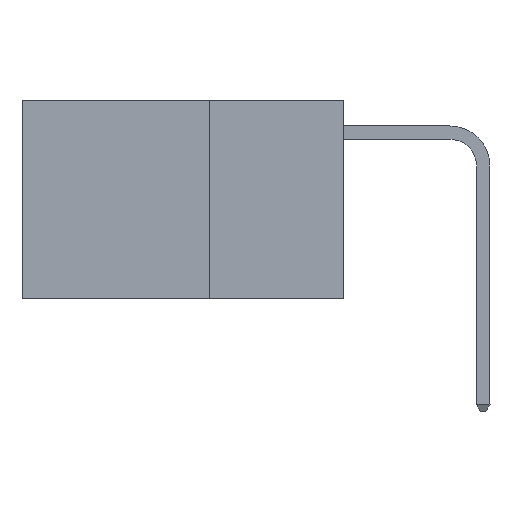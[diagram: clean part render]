
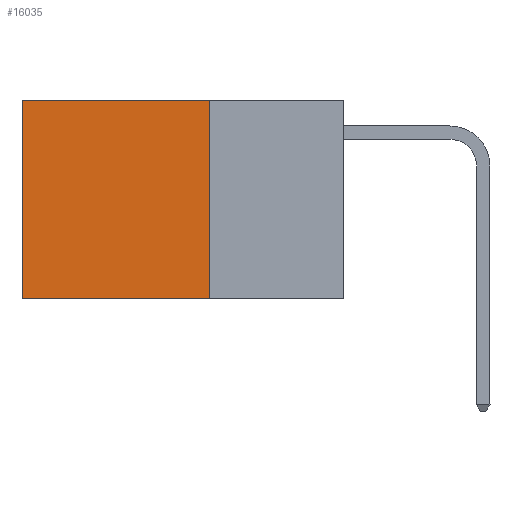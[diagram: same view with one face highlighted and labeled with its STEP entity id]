
A CAD part, left-side view. The second image highlights one B-rep face of the part: STEP entity #16035.
In plain terms, the highlighted planar face has unit normal (-1, 0, 0).
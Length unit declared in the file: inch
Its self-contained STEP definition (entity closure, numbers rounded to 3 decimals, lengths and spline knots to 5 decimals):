
#923 = EDGE_CURVE ( 'NONE', #14692, #5889, #6115, .T. ) ;
#974 = LINE ( 'NONE', #7252, #18397 ) ;
#1394 = EDGE_CURVE ( 'NONE', #14807, #5889, #8765, .T. ) ;
#2007 = DIRECTION ( 'NONE',  ( 0., 0., -1. ) ) ;
#2101 = EDGE_CURVE ( 'NONE', #15522, #14692, #974, .T. ) ;
#2105 = PLANE ( 'NONE',  #11995 ) ;
#2957 = LINE ( 'NONE', #15201, #19959 ) ;
#3341 = CARTESIAN_POINT ( 'NONE',  ( 0.2625, 0.25, -0.37 ) ) ;
#3952 = CARTESIAN_POINT ( 'NONE',  ( 0.2625, 0.6, -0.37 ) ) ;
#4254 = CARTESIAN_POINT ( 'NONE',  ( 0.2625, 0.25, -0.37 ) ) ;
#4590 = ORIENTED_EDGE ( 'NONE', *, *, #1394, .F. ) ;
#5712 = DIRECTION ( 'NONE',  ( 0., 1., 0. ) ) ;
#5859 = DIRECTION ( 'NONE',  ( 0., 0., -1. ) ) ;
#5889 = VERTEX_POINT ( 'NONE', #3952 ) ;
#6115 = LINE ( 'NONE', #16806, #12619 ) ;
#7252 = CARTESIAN_POINT ( 'NONE',  ( 0.2625, 0.25, 0. ) ) ;
#7453 = DIRECTION ( 'NONE',  ( 0., 0., -1. ) ) ;
#8116 = EDGE_CURVE ( 'NONE', #15522, #14807, #2957, .T. ) ;
#8606 = VECTOR ( 'NONE', #11951, 39.37008 ) ;
#8754 = ORIENTED_EDGE ( 'NONE', *, *, #923, .T. ) ;
#8765 = LINE ( 'NONE', #4254, #8606 ) ;
#11438 = EDGE_LOOP ( 'NONE', ( #8754, #4590, #12610, #16220 ) ) ;
#11951 = DIRECTION ( 'NONE',  ( 0., 1., 0. ) ) ;
#11995 = AXIS2_PLACEMENT_3D ( 'NONE', #19313, #19202, #2007 ) ;
#12610 = ORIENTED_EDGE ( 'NONE', *, *, #8116, .F. ) ;
#12619 = VECTOR ( 'NONE', #7453, 39.37008 ) ;
#13970 = CARTESIAN_POINT ( 'NONE',  ( 0.2625, 0.25, 0. ) ) ;
#14692 = VERTEX_POINT ( 'NONE', #17226 ) ;
#14807 = VERTEX_POINT ( 'NONE', #3341 ) ;
#15201 = CARTESIAN_POINT ( 'NONE',  ( 0.2625, 0.25, 0. ) ) ;
#15522 = VERTEX_POINT ( 'NONE', #13970 ) ;
#16035 = ADVANCED_FACE ( 'NONE', ( #16286 ), #2105, .F. ) ;
#16220 = ORIENTED_EDGE ( 'NONE', *, *, #2101, .T. ) ;
#16286 = FACE_OUTER_BOUND ( 'NONE', #11438, .T. ) ;
#16806 = CARTESIAN_POINT ( 'NONE',  ( 0.2625, 0.6, 0. ) ) ;
#17226 = CARTESIAN_POINT ( 'NONE',  ( 0.2625, 0.6, 0. ) ) ;
#18397 = VECTOR ( 'NONE', #5712, 39.37008 ) ;
#19202 = DIRECTION ( 'NONE',  ( 1., 0., 0. ) ) ;
#19313 = CARTESIAN_POINT ( 'NONE',  ( 0.2625, 0.25, 0. ) ) ;
#19959 = VECTOR ( 'NONE', #5859, 39.37008 ) ;
